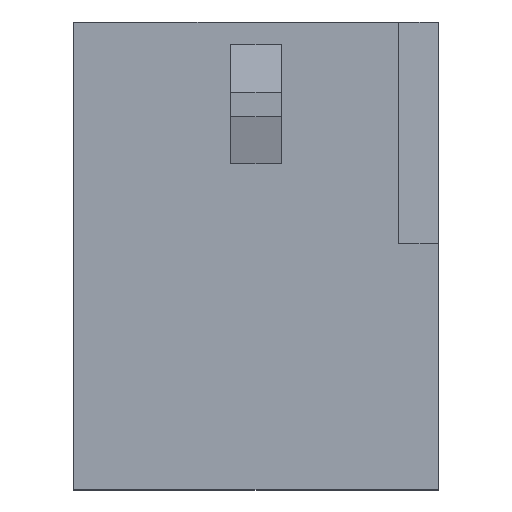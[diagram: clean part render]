
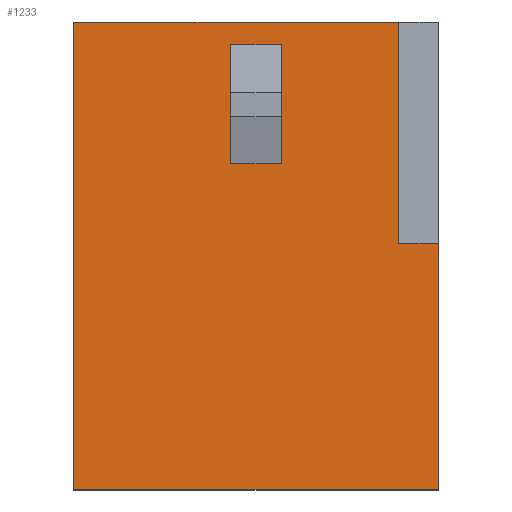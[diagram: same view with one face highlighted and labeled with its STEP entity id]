
A CAD part, top view. The second image highlights one B-rep face of the part: STEP entity #1233.
In plain terms, the highlighted planar face has unit normal (0, 0, 1).
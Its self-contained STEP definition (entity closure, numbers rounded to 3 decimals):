
#22 = LINE ( 'NONE', #2302, #1588 ) ;
#30 = ORIENTED_EDGE ( 'NONE', *, *, #223, .F. ) ;
#112 = ORIENTED_EDGE ( 'NONE', *, *, #2863, .F. ) ;
#141 = CARTESIAN_POINT ( 'NONE',  ( 7.087, 8.992, 2.54 ) ) ;
#154 = VERTEX_POINT ( 'NONE', #1291 ) ;
#178 = LINE ( 'NONE', #3453, #3951 ) ;
#223 = EDGE_CURVE ( 'NONE', #3834, #2045, #178, .T. ) ;
#325 = CARTESIAN_POINT ( 'NONE',  ( 7.087, 8.991, 2.54 ) ) ;
#513 = CARTESIAN_POINT ( 'NONE',  ( -2.324, -11.176, 2.54 ) ) ;
#514 = CARTESIAN_POINT ( 'NONE',  ( -2.324, 10.033, 2.54 ) ) ;
#529 = DIRECTION ( 'NONE',  ( -1., 0., 0. ) ) ;
#619 = EDGE_LOOP ( 'NONE', ( #3119, #1201, #30, #112 ) ) ;
#897 = CARTESIAN_POINT ( 'NONE',  ( -2.324, 0., 2.54 ) ) ;
#1051 = VERTEX_POINT ( 'NONE', #1413 ) ;
#1098 = LINE ( 'NONE', #897, #2266 ) ;
#1183 = CARTESIAN_POINT ( 'NONE',  ( 12.408, 0., 2.54 ) ) ;
#1201 = ORIENTED_EDGE ( 'NONE', *, *, #1717, .F. ) ;
#1233 = ADVANCED_FACE ( 'NONE', ( #2464, #3231 ), #4131, .T. ) ;
#1236 = EDGE_CURVE ( 'NONE', #1795, #2976, #1098, .T. ) ;
#1249 = ORIENTED_EDGE ( 'NONE', *, *, #1556, .F. ) ;
#1291 = CARTESIAN_POINT ( 'NONE',  ( 7.087, 3.608, 2.54 ) ) ;
#1377 = EDGE_CURVE ( 'NONE', #3699, #4164, #22, .T. ) ;
#1413 = CARTESIAN_POINT ( 'NONE',  ( 12.408, 10.033, 2.54 ) ) ;
#1441 = VECTOR ( 'NONE', #1981, 1000. ) ;
#1445 = LINE ( 'NONE', #3969, #3041 ) ;
#1453 = EDGE_LOOP ( 'NONE', ( #3902, #1249, #2473, #3306, #2812, #3741 ) ) ;
#1492 = VECTOR ( 'NONE', #2158, 1000. ) ;
#1517 = DIRECTION ( 'NONE',  ( 1., 0., 0. ) ) ;
#1535 = DIRECTION ( 'NONE',  ( -1., 0., 0. ) ) ;
#1556 = EDGE_CURVE ( 'NONE', #1051, #1795, #2009, .T. ) ;
#1588 = VECTOR ( 'NONE', #2590, 1000. ) ;
#1710 = LINE ( 'NONE', #4225, #1441 ) ;
#1717 = EDGE_CURVE ( 'NONE', #2045, #2367, #3186, .T. ) ;
#1731 = DIRECTION ( 'NONE',  ( 1., 0., 0. ) ) ;
#1795 = VERTEX_POINT ( 'NONE', #1183 ) ;
#1981 = DIRECTION ( 'NONE',  ( 0., 1., 0. ) ) ;
#2009 = LINE ( 'NONE', #3681, #2064 ) ;
#2017 = VECTOR ( 'NONE', #1535, 1000. ) ;
#2045 = VERTEX_POINT ( 'NONE', #2283 ) ;
#2064 = VECTOR ( 'NONE', #2980, 1000. ) ;
#2077 = CARTESIAN_POINT ( 'NONE',  ( 4.801, 8.992, 2.54 ) ) ;
#2158 = DIRECTION ( 'NONE',  ( 0., 1., 0. ) ) ;
#2170 = EDGE_CURVE ( 'NONE', #4164, #2976, #1445, .T. ) ;
#2266 = VECTOR ( 'NONE', #4185, 1000. ) ;
#2283 = CARTESIAN_POINT ( 'NONE',  ( 4.801, 8.991, 2.54 ) ) ;
#2302 = CARTESIAN_POINT ( 'NONE',  ( -2.324, -11.176, 2.54 ) ) ;
#2367 = VERTEX_POINT ( 'NONE', #2576 ) ;
#2449 = EDGE_CURVE ( 'NONE', #154, #2367, #2690, .T. ) ;
#2464 = FACE_BOUND ( 'NONE', #619, .T. ) ;
#2473 = ORIENTED_EDGE ( 'NONE', *, *, #3812, .F. ) ;
#2548 = CARTESIAN_POINT ( 'NONE',  ( 9.32, 3.608, 2.54 ) ) ;
#2576 = CARTESIAN_POINT ( 'NONE',  ( 4.801, 3.608, 2.54 ) ) ;
#2590 = DIRECTION ( 'NONE',  ( 1., 0., 0. ) ) ;
#2600 = EDGE_CURVE ( 'NONE', #3699, #3137, #1710, .T. ) ;
#2690 = LINE ( 'NONE', #2548, #2017 ) ;
#2812 = ORIENTED_EDGE ( 'NONE', *, *, #1377, .T. ) ;
#2863 = EDGE_CURVE ( 'NONE', #154, #3834, #3035, .T. ) ;
#2961 = CARTESIAN_POINT ( 'NONE',  ( -2.324, -11.176, 2.54 ) ) ;
#2976 = VERTEX_POINT ( 'NONE', #3814 ) ;
#2980 = DIRECTION ( 'NONE',  ( 0., -1., 0. ) ) ;
#3017 = CARTESIAN_POINT ( 'NONE',  ( -2.324, 10.033, 2.54 ) ) ;
#3035 = LINE ( 'NONE', #141, #1492 ) ;
#3041 = VECTOR ( 'NONE', #3607, 1000. ) ;
#3061 = DIRECTION ( 'NONE',  ( 0., -1., 0. ) ) ;
#3081 = VECTOR ( 'NONE', #3061, 1000. ) ;
#3119 = ORIENTED_EDGE ( 'NONE', *, *, #2449, .T. ) ;
#3137 = VERTEX_POINT ( 'NONE', #514 ) ;
#3186 = LINE ( 'NONE', #2077, #3081 ) ;
#3222 = VECTOR ( 'NONE', #1731, 1000. ) ;
#3231 = FACE_OUTER_BOUND ( 'NONE', #1453, .T. ) ;
#3306 = ORIENTED_EDGE ( 'NONE', *, *, #2600, .F. ) ;
#3453 = CARTESIAN_POINT ( 'NONE',  ( 9.32, 8.991, 2.54 ) ) ;
#3484 = DIRECTION ( 'NONE',  ( 0., 0., 1. ) ) ;
#3607 = DIRECTION ( 'NONE',  ( 0., 1., 0. ) ) ;
#3681 = CARTESIAN_POINT ( 'NONE',  ( 12.408, 48.54, 2.54 ) ) ;
#3699 = VERTEX_POINT ( 'NONE', #2961 ) ;
#3741 = ORIENTED_EDGE ( 'NONE', *, *, #2170, .T. ) ;
#3812 = EDGE_CURVE ( 'NONE', #3137, #1051, #4241, .T. ) ;
#3814 = CARTESIAN_POINT ( 'NONE',  ( 14.211, 0., 2.54 ) ) ;
#3834 = VERTEX_POINT ( 'NONE', #325 ) ;
#3902 = ORIENTED_EDGE ( 'NONE', *, *, #1236, .F. ) ;
#3951 = VECTOR ( 'NONE', #529, 1000. ) ;
#3969 = CARTESIAN_POINT ( 'NONE',  ( 14.211, -11.176, 2.54 ) ) ;
#4131 = PLANE ( 'NONE',  #4156 ) ;
#4156 = AXIS2_PLACEMENT_3D ( 'NONE', #513, #3484, #1517 ) ;
#4164 = VERTEX_POINT ( 'NONE', #4170 ) ;
#4170 = CARTESIAN_POINT ( 'NONE',  ( 14.211, -11.176, 2.54 ) ) ;
#4185 = DIRECTION ( 'NONE',  ( 1., 0., 0. ) ) ;
#4225 = CARTESIAN_POINT ( 'NONE',  ( -2.324, -11.176, 2.54 ) ) ;
#4241 = LINE ( 'NONE', #3017, #3222 ) ;
